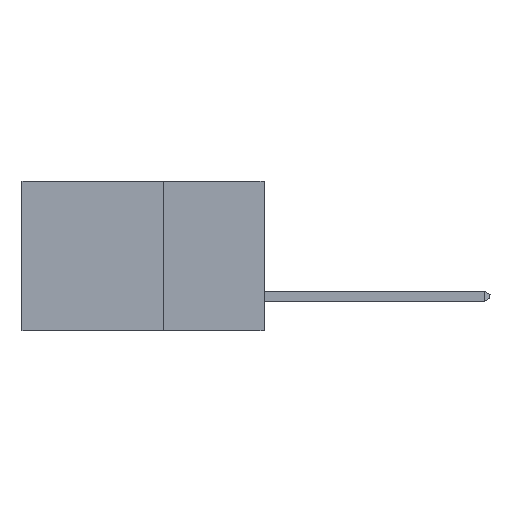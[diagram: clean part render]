
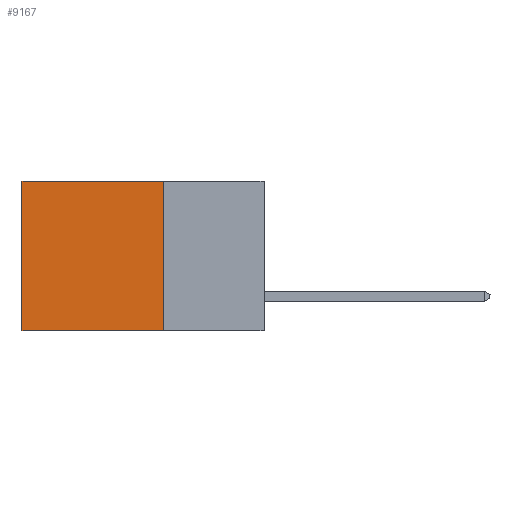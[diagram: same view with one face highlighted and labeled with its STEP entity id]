
A CAD part, left-side view. The second image highlights one B-rep face of the part: STEP entity #9167.
In plain terms, the highlighted planar face has unit normal (-1, 0, 0).
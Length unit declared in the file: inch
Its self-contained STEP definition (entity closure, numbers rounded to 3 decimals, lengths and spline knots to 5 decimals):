
#72 = LINE ( 'NONE', #3019, #5214 ) ;
#323 = VERTEX_POINT ( 'NONE', #7790 ) ;
#649 = DIRECTION ( 'NONE',  ( 0., 0., -1. ) ) ;
#656 = CARTESIAN_POINT ( 'NONE',  ( 0.298, 0.25, 0. ) ) ;
#979 = DIRECTION ( 'NONE',  ( 0., 0., -1. ) ) ;
#1303 = VERTEX_POINT ( 'NONE', #9138 ) ;
#1358 = EDGE_CURVE ( 'NONE', #1303, #8592, #10922, .T. ) ;
#1724 = VECTOR ( 'NONE', #979, 39.37008 ) ;
#2209 = DIRECTION ( 'NONE',  ( 0., 0., -1. ) ) ;
#3019 = CARTESIAN_POINT ( 'NONE',  ( 0.298, 0.25, 0. ) ) ;
#3500 = ORIENTED_EDGE ( 'NONE', *, *, #6334, .T. ) ;
#3759 = FACE_OUTER_BOUND ( 'NONE', #6677, .T. ) ;
#3811 = ORIENTED_EDGE ( 'NONE', *, *, #4836, .F. ) ;
#3945 = LINE ( 'NONE', #6840, #1724 ) ;
#4119 = CARTESIAN_POINT ( 'NONE',  ( 0.298, 0.25, 0. ) ) ;
#4836 = EDGE_CURVE ( 'NONE', #5662, #1303, #72, .T. ) ;
#4981 = CARTESIAN_POINT ( 'NONE',  ( 0.298, 0.25, -0.37 ) ) ;
#4982 = AXIS2_PLACEMENT_3D ( 'NONE', #10819, #8270, #649 ) ;
#5174 = VECTOR ( 'NONE', #5670, 39.37008 ) ;
#5214 = VECTOR ( 'NONE', #2209, 39.37008 ) ;
#5443 = LINE ( 'NONE', #656, #5174 ) ;
#5662 = VERTEX_POINT ( 'NONE', #4119 ) ;
#5670 = DIRECTION ( 'NONE',  ( 0., 1., 0. ) ) ;
#6334 = EDGE_CURVE ( 'NONE', #323, #8592, #3945, .T. ) ;
#6677 = EDGE_LOOP ( 'NONE', ( #3500, #8681, #3811, #10025 ) ) ;
#6820 = DIRECTION ( 'NONE',  ( 0., 1., 0. ) ) ;
#6840 = CARTESIAN_POINT ( 'NONE',  ( 0.298, 0.6, 0. ) ) ;
#7790 = CARTESIAN_POINT ( 'NONE',  ( 0.298, 0.6, 0. ) ) ;
#7915 = EDGE_CURVE ( 'NONE', #5662, #323, #5443, .T. ) ;
#8270 = DIRECTION ( 'NONE',  ( 1., 0., 0. ) ) ;
#8592 = VERTEX_POINT ( 'NONE', #10404 ) ;
#8681 = ORIENTED_EDGE ( 'NONE', *, *, #1358, .F. ) ;
#9138 = CARTESIAN_POINT ( 'NONE',  ( 0.298, 0.25, -0.37 ) ) ;
#9167 = ADVANCED_FACE ( 'NONE', ( #3759 ), #9978, .F. ) ;
#9978 = PLANE ( 'NONE',  #4982 ) ;
#10025 = ORIENTED_EDGE ( 'NONE', *, *, #7915, .T. ) ;
#10404 = CARTESIAN_POINT ( 'NONE',  ( 0.298, 0.6, -0.37 ) ) ;
#10666 = VECTOR ( 'NONE', #6820, 39.37008 ) ;
#10819 = CARTESIAN_POINT ( 'NONE',  ( 0.298, 0.25, 0. ) ) ;
#10922 = LINE ( 'NONE', #4981, #10666 ) ;
